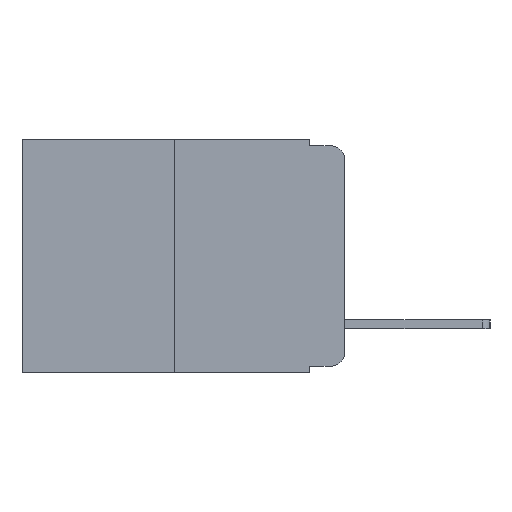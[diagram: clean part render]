
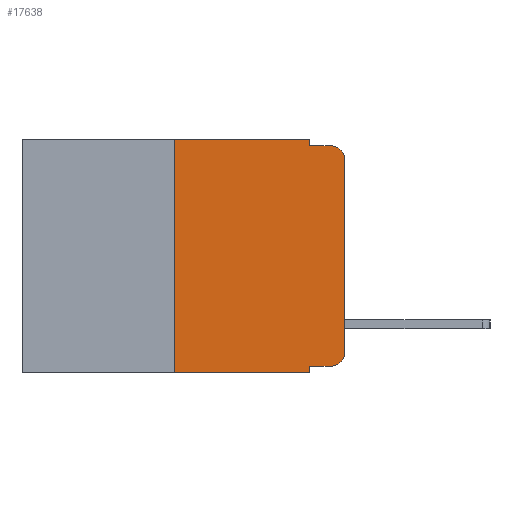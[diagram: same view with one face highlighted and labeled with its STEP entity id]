
A CAD part, left-side view. The second image highlights one B-rep face of the part: STEP entity #17638.
In plain terms, the highlighted planar face has unit normal (-1, 0, 0).
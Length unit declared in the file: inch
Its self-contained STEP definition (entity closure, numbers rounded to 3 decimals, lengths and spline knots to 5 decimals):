
#34 = VERTEX_POINT ( 'NONE', #10054 ) ;
#531 = DIRECTION ( 'NONE',  ( 0., -1., 0. ) ) ;
#538 = VERTEX_POINT ( 'NONE', #16744 ) ;
#618 = EDGE_CURVE ( 'NONE', #2145, #13045, #3526, .T. ) ;
#1099 = DIRECTION ( 'NONE',  ( 0., 0., -1. ) ) ;
#1307 = DIRECTION ( 'NONE',  ( 0., 0., -1. ) ) ;
#1390 = LINE ( 'NONE', #8133, #15826 ) ;
#1425 = VERTEX_POINT ( 'NONE', #12703 ) ;
#2145 = VERTEX_POINT ( 'NONE', #4667 ) ;
#2218 = LINE ( 'NONE', #15153, #13352 ) ;
#2514 = AXIS2_PLACEMENT_3D ( 'NONE', #18302, #11986, #12004 ) ;
#2585 = EDGE_CURVE ( 'NONE', #17073, #4912, #3666, .T. ) ;
#2670 = LINE ( 'NONE', #13154, #3121 ) ;
#3002 = DIRECTION ( 'NONE',  ( 0., -1., 0. ) ) ;
#3121 = VECTOR ( 'NONE', #3002, 39.37008 ) ;
#3526 = CIRCLE ( 'NONE', #2514, 0.02 ) ;
#3637 = DIRECTION ( 'NONE',  ( 0., 0., 1. ) ) ;
#3666 = CIRCLE ( 'NONE', #17699, 0.02 ) ;
#4043 = CARTESIAN_POINT ( 'NONE',  ( 0., 0.473, 0. ) ) ;
#4449 = LINE ( 'NONE', #7742, #15505 ) ;
#4667 = CARTESIAN_POINT ( 'NONE',  ( 0., 0.02, -0.333 ) ) ;
#4786 = CARTESIAN_POINT ( 'NONE',  ( 0., 0.051, -0.333 ) ) ;
#4912 = VERTEX_POINT ( 'NONE', #13492 ) ;
#5189 = CARTESIAN_POINT ( 'NONE',  ( 0., 0.051, -0.333 ) ) ;
#5202 = VECTOR ( 'NONE', #12806, 39.37008 ) ;
#5549 = VERTEX_POINT ( 'NONE', #4786 ) ;
#5578 = DIRECTION ( 'NONE',  ( 1., 0., 0. ) ) ;
#5621 = ORIENTED_EDGE ( 'NONE', *, *, #11983, .T. ) ;
#5839 = VERTEX_POINT ( 'NONE', #15498 ) ;
#6393 = CARTESIAN_POINT ( 'NONE',  ( 0., 0.25, 0. ) ) ;
#7715 = EDGE_CURVE ( 'NONE', #5549, #2145, #16753, .T. ) ;
#7742 = CARTESIAN_POINT ( 'NONE',  ( 0., 0.473, 0. ) ) ;
#8133 = CARTESIAN_POINT ( 'NONE',  ( 0., 0.051, 0. ) ) ;
#8426 = EDGE_LOOP ( 'NONE', ( #16399, #17260, #17710, #11073, #15758, #16191, #5621, #9533, #17936, #18359 ) ) ;
#9037 = CARTESIAN_POINT ( 'NONE',  ( 0., 0.25, 0. ) ) ;
#9533 = ORIENTED_EDGE ( 'NONE', *, *, #17018, .F. ) ;
#10054 = CARTESIAN_POINT ( 'NONE',  ( 0., 0.051, 0. ) ) ;
#10155 = CARTESIAN_POINT ( 'NONE',  ( 0., 0., -0.03 ) ) ;
#10166 = EDGE_CURVE ( 'NONE', #538, #15028, #12301, .T. ) ;
#10467 = DIRECTION ( 'NONE',  ( 0., 0., 1. ) ) ;
#11073 = ORIENTED_EDGE ( 'NONE', *, *, #16801, .F. ) ;
#11148 = EDGE_CURVE ( 'NONE', #1425, #4912, #12922, .T. ) ;
#11372 = CARTESIAN_POINT ( 'NONE',  ( 0., 0.051, -0.01 ) ) ;
#11822 = VECTOR ( 'NONE', #1307, 39.37008 ) ;
#11845 = VECTOR ( 'NONE', #10467, 39.37008 ) ;
#11983 = EDGE_CURVE ( 'NONE', #538, #5839, #2670, .T. ) ;
#11986 = DIRECTION ( 'NONE',  ( -1., 0., 0. ) ) ;
#12004 = DIRECTION ( 'NONE',  ( 0., 0., -1. ) ) ;
#12301 = LINE ( 'NONE', #9037, #11845 ) ;
#12703 = CARTESIAN_POINT ( 'NONE',  ( 0., 0.051, -0.01 ) ) ;
#12806 = DIRECTION ( 'NONE',  ( 0., -1., 0. ) ) ;
#12807 = PLANE ( 'NONE',  #16562 ) ;
#12917 = FACE_OUTER_BOUND ( 'NONE', #8426, .T. ) ;
#12922 = LINE ( 'NONE', #11372, #5202 ) ;
#12951 = EDGE_CURVE ( 'NONE', #15028, #34, #4449, .T. ) ;
#13045 = VERTEX_POINT ( 'NONE', #17876 ) ;
#13154 = CARTESIAN_POINT ( 'NONE',  ( 0., 0.473, -0.343 ) ) ;
#13352 = VECTOR ( 'NONE', #3637, 39.37008 ) ;
#13357 = CARTESIAN_POINT ( 'NONE',  ( 0., 0.02, -0.03 ) ) ;
#13478 = VECTOR ( 'NONE', #16672, 39.37008 ) ;
#13492 = CARTESIAN_POINT ( 'NONE',  ( 0., 0.02, -0.01 ) ) ;
#13851 = DIRECTION ( 'NONE',  ( -1., 0., 0. ) ) ;
#15028 = VERTEX_POINT ( 'NONE', #6393 ) ;
#15153 = CARTESIAN_POINT ( 'NONE',  ( 0., 0., 0. ) ) ;
#15498 = CARTESIAN_POINT ( 'NONE',  ( 0., 0.051, -0.343 ) ) ;
#15505 = VECTOR ( 'NONE', #531, 39.37008 ) ;
#15598 = LINE ( 'NONE', #18466, #11822 ) ;
#15652 = DIRECTION ( 'NONE',  ( 0., 0., -1. ) ) ;
#15758 = ORIENTED_EDGE ( 'NONE', *, *, #12951, .F. ) ;
#15826 = VECTOR ( 'NONE', #18060, 39.37008 ) ;
#16191 = ORIENTED_EDGE ( 'NONE', *, *, #10166, .F. ) ;
#16399 = ORIENTED_EDGE ( 'NONE', *, *, #18055, .T. ) ;
#16562 = AXIS2_PLACEMENT_3D ( 'NONE', #4043, #5578, #15652 ) ;
#16672 = DIRECTION ( 'NONE',  ( 0., -1., 0. ) ) ;
#16744 = CARTESIAN_POINT ( 'NONE',  ( 0., 0.25, -0.343 ) ) ;
#16753 = LINE ( 'NONE', #5189, #13478 ) ;
#16801 = EDGE_CURVE ( 'NONE', #34, #1425, #1390, .T. ) ;
#17018 = EDGE_CURVE ( 'NONE', #5549, #5839, #15598, .T. ) ;
#17073 = VERTEX_POINT ( 'NONE', #10155 ) ;
#17260 = ORIENTED_EDGE ( 'NONE', *, *, #2585, .T. ) ;
#17638 = ADVANCED_FACE ( 'NONE', ( #12917 ), #12807, .F. ) ;
#17699 = AXIS2_PLACEMENT_3D ( 'NONE', #13357, #13851, #1099 ) ;
#17710 = ORIENTED_EDGE ( 'NONE', *, *, #11148, .F. ) ;
#17876 = CARTESIAN_POINT ( 'NONE',  ( 0., 0., -0.313 ) ) ;
#17936 = ORIENTED_EDGE ( 'NONE', *, *, #7715, .T. ) ;
#18055 = EDGE_CURVE ( 'NONE', #13045, #17073, #2218, .T. ) ;
#18060 = DIRECTION ( 'NONE',  ( 0., 0., -1. ) ) ;
#18302 = CARTESIAN_POINT ( 'NONE',  ( 0., 0.02, -0.313 ) ) ;
#18359 = ORIENTED_EDGE ( 'NONE', *, *, #618, .T. ) ;
#18466 = CARTESIAN_POINT ( 'NONE',  ( 0., 0.051, 0. ) ) ;
